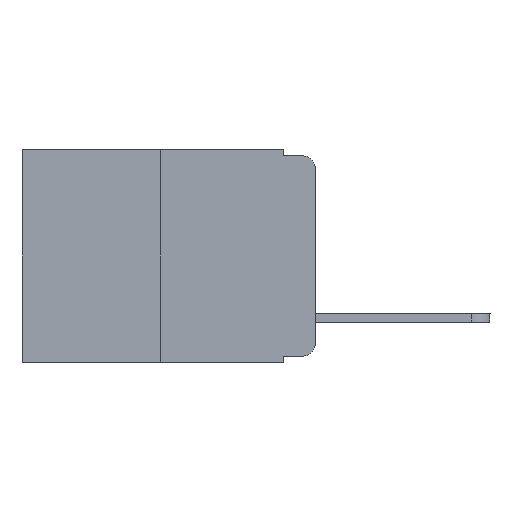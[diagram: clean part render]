
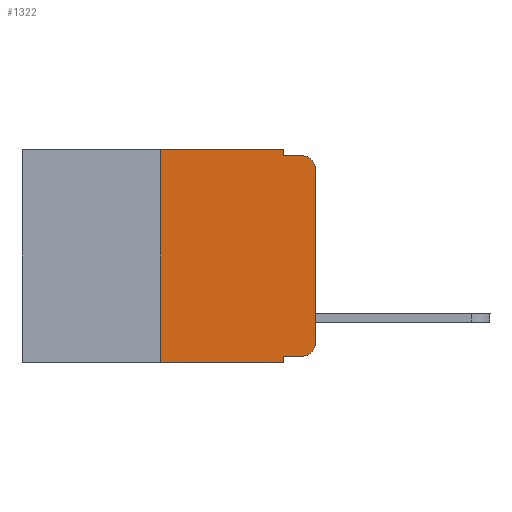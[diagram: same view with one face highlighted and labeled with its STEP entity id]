
A CAD part, left-side view. The second image highlights one B-rep face of the part: STEP entity #1322.
In plain terms, the highlighted planar face has unit normal (-1, 0, 0).
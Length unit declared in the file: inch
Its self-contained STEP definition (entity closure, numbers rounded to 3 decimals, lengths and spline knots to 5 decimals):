
#70 = LINE ( 'NONE', #5713, #4863 ) ;
#154 = LINE ( 'NONE', #15314, #13983 ) ;
#220 = DIRECTION ( 'NONE',  ( 0., 0., -1. ) ) ;
#240 = VERTEX_POINT ( 'NONE', #15784 ) ;
#262 = VERTEX_POINT ( 'NONE', #3747 ) ;
#779 = EDGE_CURVE ( 'NONE', #240, #13100, #8696, .T. ) ;
#912 = VERTEX_POINT ( 'NONE', #5432 ) ;
#1322 = ADVANCED_FACE ( 'NONE', ( #10827 ), #11102, .F. ) ;
#1400 = DIRECTION ( 'NONE',  ( 0., -1., 0. ) ) ;
#1444 = DIRECTION ( 'NONE',  ( 0., -1., 0. ) ) ;
#1605 = VERTEX_POINT ( 'NONE', #9580 ) ;
#1880 = LINE ( 'NONE', #8664, #11261 ) ;
#1905 = CARTESIAN_POINT ( 'NONE',  ( 0., 0.051, 0. ) ) ;
#2057 = EDGE_CURVE ( 'NONE', #262, #10571, #154, .T. ) ;
#2532 = ORIENTED_EDGE ( 'NONE', *, *, #2768, .F. ) ;
#2654 = LINE ( 'NONE', #8102, #3478 ) ;
#2658 = DIRECTION ( 'NONE',  ( -1., 0., 0. ) ) ;
#2736 = DIRECTION ( 'NONE',  ( 0., 0., 1. ) ) ;
#2753 = CARTESIAN_POINT ( 'NONE',  ( 0., 0., -0.313 ) ) ;
#2768 = EDGE_CURVE ( 'NONE', #5340, #13100, #1880, .T. ) ;
#2908 = CARTESIAN_POINT ( 'NONE',  ( 0., 0.473, 0. ) ) ;
#3088 = DIRECTION ( 'NONE',  ( 0., 0., -1. ) ) ;
#3478 = VECTOR ( 'NONE', #2736, 39.37008 ) ;
#3747 = CARTESIAN_POINT ( 'NONE',  ( 0., 0.25, 0. ) ) ;
#3809 = EDGE_CURVE ( 'NONE', #912, #4852, #6711, .T. ) ;
#4245 = CARTESIAN_POINT ( 'NONE',  ( 0., 0.051, 0. ) ) ;
#4419 = AXIS2_PLACEMENT_3D ( 'NONE', #15937, #2658, #9443 ) ;
#4506 = CARTESIAN_POINT ( 'NONE',  ( 0., 0.02, -0.313 ) ) ;
#4648 = DIRECTION ( 'NONE',  ( 0., -1., 0. ) ) ;
#4668 = CARTESIAN_POINT ( 'NONE',  ( 0., 0.25, -0.343 ) ) ;
#4852 = VERTEX_POINT ( 'NONE', #8714 ) ;
#4863 = VECTOR ( 'NONE', #17562, 39.37008 ) ;
#5323 = EDGE_LOOP ( 'NONE', ( #7920, #5474, #2532, #5582, #8895, #11997, #13469, #5894, #14290, #14411 ) ) ;
#5340 = VERTEX_POINT ( 'NONE', #8845 ) ;
#5432 = CARTESIAN_POINT ( 'NONE',  ( 0., 0.051, -0.333 ) ) ;
#5474 = ORIENTED_EDGE ( 'NONE', *, *, #779, .T. ) ;
#5582 = ORIENTED_EDGE ( 'NONE', *, *, #13749, .F. ) ;
#5713 = CARTESIAN_POINT ( 'NONE',  ( 0., 0.051, 0. ) ) ;
#5894 = ORIENTED_EDGE ( 'NONE', *, *, #9284, .F. ) ;
#5930 = DIRECTION ( 'NONE',  ( 0., 0., -1. ) ) ;
#5936 = EDGE_CURVE ( 'NONE', #8188, #262, #11456, .T. ) ;
#6711 = LINE ( 'NONE', #17583, #9295 ) ;
#7920 = ORIENTED_EDGE ( 'NONE', *, *, #15381, .T. ) ;
#7940 = EDGE_CURVE ( 'NONE', #8188, #1605, #17411, .T. ) ;
#8102 = CARTESIAN_POINT ( 'NONE',  ( 0., 0., 0. ) ) ;
#8188 = VERTEX_POINT ( 'NONE', #4668 ) ;
#8204 = VECTOR ( 'NONE', #5930, 39.37008 ) ;
#8442 = DIRECTION ( 'NONE',  ( -1., 0., 0. ) ) ;
#8536 = AXIS2_PLACEMENT_3D ( 'NONE', #2908, #12432, #220 ) ;
#8664 = CARTESIAN_POINT ( 'NONE',  ( 0., 0.051, -0.01 ) ) ;
#8696 = CIRCLE ( 'NONE', #4419, 0.02 ) ;
#8714 = CARTESIAN_POINT ( 'NONE',  ( 0., 0.02, -0.333 ) ) ;
#8845 = CARTESIAN_POINT ( 'NONE',  ( 0., 0.051, -0.01 ) ) ;
#8895 = ORIENTED_EDGE ( 'NONE', *, *, #2057, .F. ) ;
#9284 = EDGE_CURVE ( 'NONE', #912, #1605, #14188, .T. ) ;
#9295 = VECTOR ( 'NONE', #11938, 39.37008 ) ;
#9301 = CARTESIAN_POINT ( 'NONE',  ( 0., 0.02, -0.01 ) ) ;
#9443 = DIRECTION ( 'NONE',  ( 0., 0., -1. ) ) ;
#9580 = CARTESIAN_POINT ( 'NONE',  ( 0., 0.051, -0.343 ) ) ;
#10356 = AXIS2_PLACEMENT_3D ( 'NONE', #4506, #8442, #3088 ) ;
#10571 = VERTEX_POINT ( 'NONE', #4245 ) ;
#10800 = CARTESIAN_POINT ( 'NONE',  ( 0., 0.473, -0.343 ) ) ;
#10827 = FACE_OUTER_BOUND ( 'NONE', #5323, .T. ) ;
#11102 = PLANE ( 'NONE',  #8536 ) ;
#11261 = VECTOR ( 'NONE', #4648, 39.37008 ) ;
#11456 = LINE ( 'NONE', #14045, #12400 ) ;
#11938 = DIRECTION ( 'NONE',  ( 0., -1., 0. ) ) ;
#11997 = ORIENTED_EDGE ( 'NONE', *, *, #5936, .F. ) ;
#12380 = VERTEX_POINT ( 'NONE', #2753 ) ;
#12400 = VECTOR ( 'NONE', #15472, 39.37008 ) ;
#12432 = DIRECTION ( 'NONE',  ( 1., 0., 0. ) ) ;
#13100 = VERTEX_POINT ( 'NONE', #9301 ) ;
#13469 = ORIENTED_EDGE ( 'NONE', *, *, #7940, .T. ) ;
#13533 = VECTOR ( 'NONE', #1444, 39.37008 ) ;
#13749 = EDGE_CURVE ( 'NONE', #10571, #5340, #70, .T. ) ;
#13983 = VECTOR ( 'NONE', #1400, 39.37008 ) ;
#14045 = CARTESIAN_POINT ( 'NONE',  ( 0., 0.25, 0. ) ) ;
#14188 = LINE ( 'NONE', #1905, #8204 ) ;
#14290 = ORIENTED_EDGE ( 'NONE', *, *, #3809, .T. ) ;
#14411 = ORIENTED_EDGE ( 'NONE', *, *, #15846, .T. ) ;
#15314 = CARTESIAN_POINT ( 'NONE',  ( 0., 0.473, 0. ) ) ;
#15381 = EDGE_CURVE ( 'NONE', #12380, #240, #2654, .T. ) ;
#15472 = DIRECTION ( 'NONE',  ( 0., 0., 1. ) ) ;
#15784 = CARTESIAN_POINT ( 'NONE',  ( 0., 0., -0.03 ) ) ;
#15846 = EDGE_CURVE ( 'NONE', #4852, #12380, #16920, .T. ) ;
#15937 = CARTESIAN_POINT ( 'NONE',  ( 0., 0.02, -0.03 ) ) ;
#16920 = CIRCLE ( 'NONE', #10356, 0.02 ) ;
#17411 = LINE ( 'NONE', #10800, #13533 ) ;
#17562 = DIRECTION ( 'NONE',  ( 0., 0., -1. ) ) ;
#17583 = CARTESIAN_POINT ( 'NONE',  ( 0., 0.051, -0.333 ) ) ;
